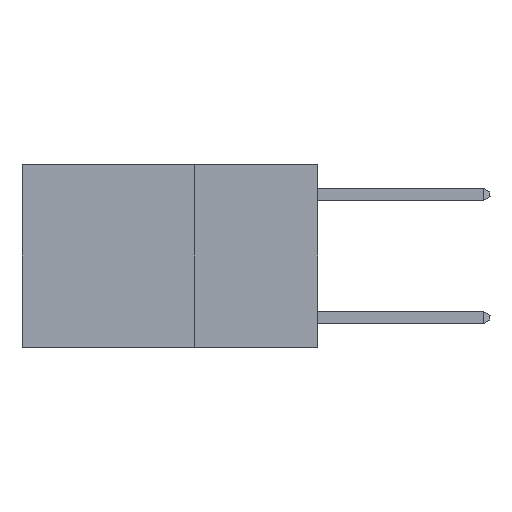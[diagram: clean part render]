
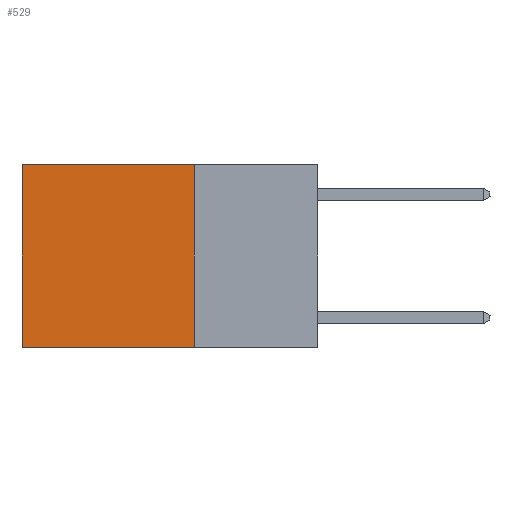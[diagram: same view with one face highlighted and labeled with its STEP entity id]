
A CAD part, left-side view. The second image highlights one B-rep face of the part: STEP entity #529.
In plain terms, the highlighted planar face has unit normal (-1, 0, 0).
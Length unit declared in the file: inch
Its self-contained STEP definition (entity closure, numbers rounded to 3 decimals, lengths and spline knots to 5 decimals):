
#529 = ADVANCED_FACE ( 'NONE', ( #1110 ), #14548, .F. ) ;
#893 = EDGE_LOOP ( 'NONE', ( #6211, #9736, #15080, #6485 ) ) ;
#1110 = FACE_OUTER_BOUND ( 'NONE', #893, .T. ) ;
#1352 = DIRECTION ( 'NONE',  ( 0., 0., -1. ) ) ;
#1432 = DIRECTION ( 'NONE',  ( 1., 0., 0. ) ) ;
#1566 = VERTEX_POINT ( 'NONE', #10058 ) ;
#1634 = VECTOR ( 'NONE', #2130, 39.37008 ) ;
#2130 = DIRECTION ( 'NONE',  ( 0., 0., -1. ) ) ;
#3684 = CARTESIAN_POINT ( 'NONE',  ( 0.2625, 0.25, -0.37 ) ) ;
#5247 = AXIS2_PLACEMENT_3D ( 'NONE', #11051, #1432, #1352 ) ;
#5672 = CARTESIAN_POINT ( 'NONE',  ( 0.2625, 0.25, -0.37 ) ) ;
#6009 = CARTESIAN_POINT ( 'NONE',  ( 0.2625, 0.25, 0. ) ) ;
#6211 = ORIENTED_EDGE ( 'NONE', *, *, #12882, .T. ) ;
#6485 = ORIENTED_EDGE ( 'NONE', *, *, #11933, .T. ) ;
#8034 = EDGE_CURVE ( 'NONE', #12488, #8603, #15336, .T. ) ;
#8081 = CARTESIAN_POINT ( 'NONE',  ( 0.2625, 0.25, 0. ) ) ;
#8087 = LINE ( 'NONE', #8293, #1634 ) ;
#8293 = CARTESIAN_POINT ( 'NONE',  ( 0.2625, 0.6, 0. ) ) ;
#8326 = DIRECTION ( 'NONE',  ( 0., 1., 0. ) ) ;
#8603 = VERTEX_POINT ( 'NONE', #3684 ) ;
#9007 = VECTOR ( 'NONE', #9333, 39.37008 ) ;
#9307 = LINE ( 'NONE', #14258, #13796 ) ;
#9333 = DIRECTION ( 'NONE',  ( 0., 1., 0. ) ) ;
#9736 = ORIENTED_EDGE ( 'NONE', *, *, #14591, .F. ) ;
#10058 = CARTESIAN_POINT ( 'NONE',  ( 0.2625, 0.6, -0.37 ) ) ;
#11051 = CARTESIAN_POINT ( 'NONE',  ( 0.2625, 0.25, 0. ) ) ;
#11836 = VECTOR ( 'NONE', #12827, 39.37008 ) ;
#11933 = EDGE_CURVE ( 'NONE', #12488, #14250, #9307, .T. ) ;
#12488 = VERTEX_POINT ( 'NONE', #6009 ) ;
#12815 = LINE ( 'NONE', #5672, #9007 ) ;
#12827 = DIRECTION ( 'NONE',  ( 0., 0., -1. ) ) ;
#12882 = EDGE_CURVE ( 'NONE', #14250, #1566, #8087, .T. ) ;
#12900 = CARTESIAN_POINT ( 'NONE',  ( 0.2625, 0.6, 0. ) ) ;
#13796 = VECTOR ( 'NONE', #8326, 39.37008 ) ;
#14250 = VERTEX_POINT ( 'NONE', #12900 ) ;
#14258 = CARTESIAN_POINT ( 'NONE',  ( 0.2625, 0.25, 0. ) ) ;
#14548 = PLANE ( 'NONE',  #5247 ) ;
#14591 = EDGE_CURVE ( 'NONE', #8603, #1566, #12815, .T. ) ;
#15080 = ORIENTED_EDGE ( 'NONE', *, *, #8034, .F. ) ;
#15336 = LINE ( 'NONE', #8081, #11836 ) ;
